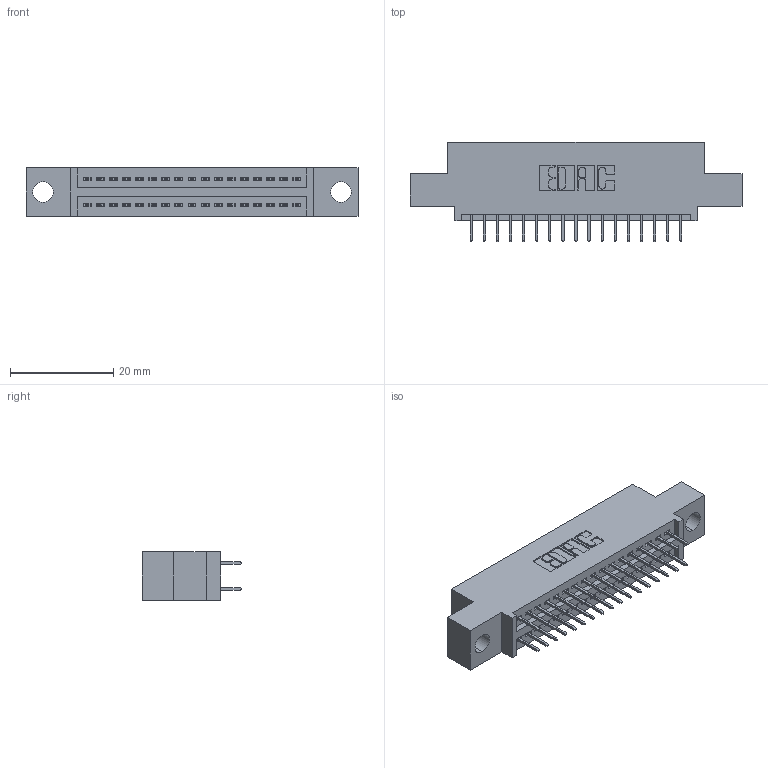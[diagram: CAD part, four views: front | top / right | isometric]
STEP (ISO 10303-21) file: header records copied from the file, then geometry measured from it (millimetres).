
FILE_DESCRIPTION (( 'STEP AP203' ), '1' );
FILE_NAME ('345-034-524-504.STEP', '2021-05-20T00:02:04', ( '' ), ( '' ), 'SwSTEP 2.0', 'SolidWorks 2020', '' );
FILE_SCHEMA (( 'CONFIG_CONTROL_DESIGN' ));
Length unit declared in the file: inch
Products named in the file (3): 345 Part_0.110 Offset - 0.156 Dia-TI; 345-292-001_345-293-124; 345-034-524-504
Assembly tree (35 placements, depth 2):
  345-034-524-504
    345 Part_0.110 Offset - 0.156 Dia-TI
    345-292-001_345-293-124  x34
Bounding box: 64.39 x 19.35 x 9.4 mm (x, y, z)
Volume: 5792 mm3; surface area: 7885.9 mm2
Topology: 35 solids, 35 shells, 1980 faces, 5591 edges, 3590 vertices
Faces by surface type: plane 1424, cylinder 556
Entity records: 17329 total; most frequent: CARTESIAN_POINT 2934, ORIENTED_EDGE 2866, DIRECTION 2617, EDGE_CURVE 1433, VECTOR 1237, LINE 1237, VERTEX_POINT 950, AXIS2_PLACEMENT_3D 690
